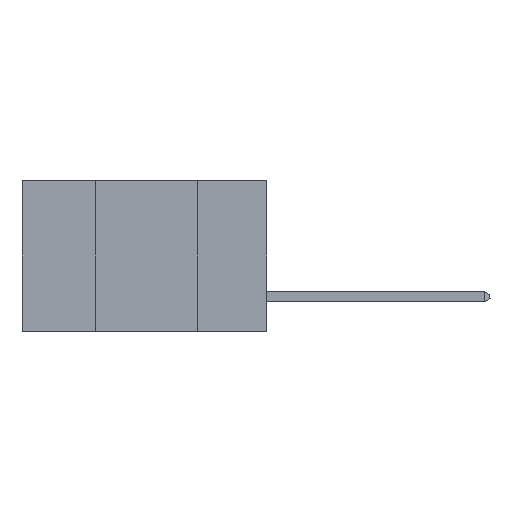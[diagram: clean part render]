
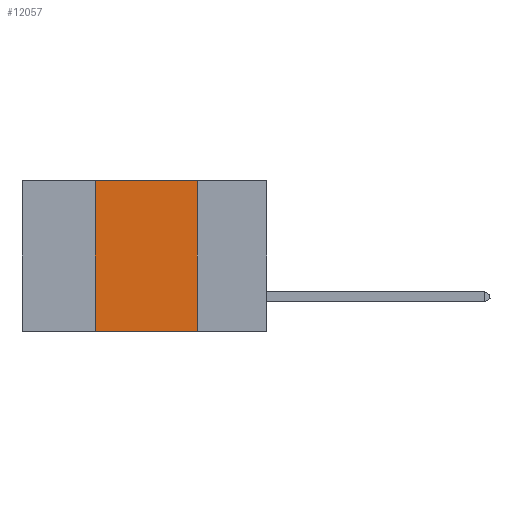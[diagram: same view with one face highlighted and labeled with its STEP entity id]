
A CAD part, left-side view. The second image highlights one B-rep face of the part: STEP entity #12057.
In plain terms, the highlighted planar face has unit normal (-1, 0, 0).
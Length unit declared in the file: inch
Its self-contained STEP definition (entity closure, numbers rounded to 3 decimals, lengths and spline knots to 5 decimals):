
#551 = EDGE_LOOP ( 'NONE', ( #3503, #15102, #13409, #19477 ) ) ;
#1851 = AXIS2_PLACEMENT_3D ( 'NONE', #9710, #3761, #7832 ) ;
#1898 = CARTESIAN_POINT ( 'NONE',  ( 0., 0.17, 0. ) ) ;
#2500 = FACE_OUTER_BOUND ( 'NONE', #551, .T. ) ;
#3503 = ORIENTED_EDGE ( 'NONE', *, *, #24323, .F. ) ;
#3761 = DIRECTION ( 'NONE',  ( 1., 0., 0. ) ) ;
#4331 = VERTEX_POINT ( 'NONE', #1898 ) ;
#4674 = CARTESIAN_POINT ( 'NONE',  ( 0., 0.17, -0.37 ) ) ;
#5650 = VECTOR ( 'NONE', #26022, 39.37008 ) ;
#6696 = VERTEX_POINT ( 'NONE', #23269 ) ;
#7565 = VERTEX_POINT ( 'NONE', #17983 ) ;
#7832 = DIRECTION ( 'NONE',  ( 0., 0., -1. ) ) ;
#8952 = VECTOR ( 'NONE', #24698, 39.37008 ) ;
#9710 = CARTESIAN_POINT ( 'NONE',  ( 0., 0.6, 0. ) ) ;
#11240 = EDGE_CURVE ( 'NONE', #6696, #20801, #17445, .T. ) ;
#12057 = ADVANCED_FACE ( 'NONE', ( #2500 ), #20005, .F. ) ;
#13409 = ORIENTED_EDGE ( 'NONE', *, *, #23492, .F. ) ;
#14011 = VECTOR ( 'NONE', #23829, 39.37008 ) ;
#15102 = ORIENTED_EDGE ( 'NONE', *, *, #23860, .F. ) ;
#15655 = DIRECTION ( 'NONE',  ( 0., -1., 0. ) ) ;
#15938 = VECTOR ( 'NONE', #15655, 39.37008 ) ;
#15959 = LINE ( 'NONE', #19810, #14011 ) ;
#16410 = CARTESIAN_POINT ( 'NONE',  ( 0., 0.6, 0. ) ) ;
#17445 = LINE ( 'NONE', #21993, #5650 ) ;
#17844 = LINE ( 'NONE', #16410, #15938 ) ;
#17983 = CARTESIAN_POINT ( 'NONE',  ( 0., 0.42, 0. ) ) ;
#19477 = ORIENTED_EDGE ( 'NONE', *, *, #11240, .T. ) ;
#19810 = CARTESIAN_POINT ( 'NONE',  ( 0., 0.42, 0. ) ) ;
#20005 = PLANE ( 'NONE',  #1851 ) ;
#20801 = VERTEX_POINT ( 'NONE', #4674 ) ;
#21993 = CARTESIAN_POINT ( 'NONE',  ( 0., 0.6, -0.37 ) ) ;
#23269 = CARTESIAN_POINT ( 'NONE',  ( 0., 0.42, -0.37 ) ) ;
#23492 = EDGE_CURVE ( 'NONE', #6696, #7565, #15959, .T. ) ;
#23829 = DIRECTION ( 'NONE',  ( 0., 0., 1. ) ) ;
#23860 = EDGE_CURVE ( 'NONE', #7565, #4331, #17844, .T. ) ;
#24111 = LINE ( 'NONE', #25249, #8952 ) ;
#24323 = EDGE_CURVE ( 'NONE', #4331, #20801, #24111, .T. ) ;
#24698 = DIRECTION ( 'NONE',  ( 0., 0., -1. ) ) ;
#25249 = CARTESIAN_POINT ( 'NONE',  ( 0., 0.17, 0. ) ) ;
#26022 = DIRECTION ( 'NONE',  ( 0., -1., 0. ) ) ;
